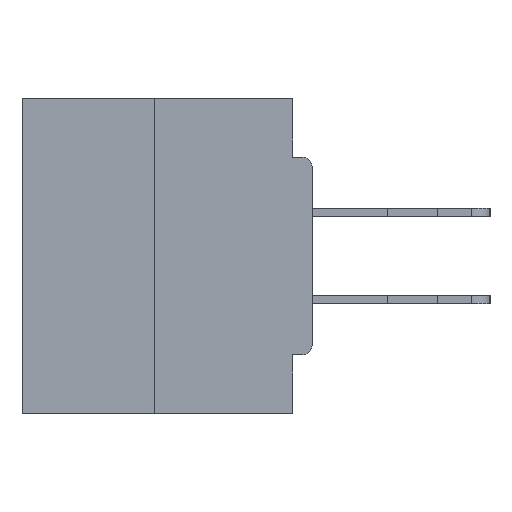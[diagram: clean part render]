
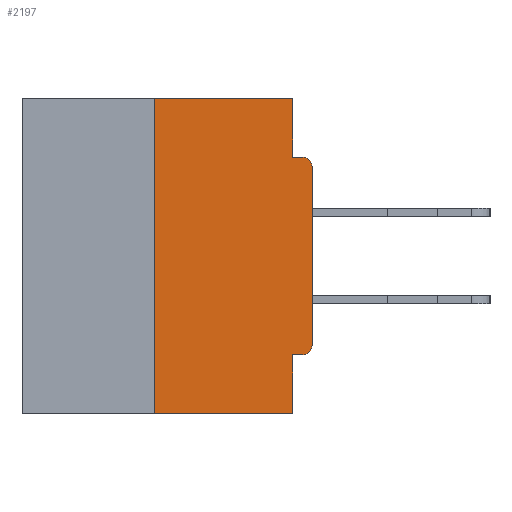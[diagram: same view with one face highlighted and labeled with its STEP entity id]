
A CAD part, left-side view. The second image highlights one B-rep face of the part: STEP entity #2197.
In plain terms, the highlighted planar face has unit normal (-1, 0, 0).
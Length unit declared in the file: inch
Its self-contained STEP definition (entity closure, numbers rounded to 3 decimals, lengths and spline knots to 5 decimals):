
#971 = EDGE_CURVE ( 'NONE', #14199, #31464, #19182, .T. ) ;
#2197 = ADVANCED_FACE ( 'NONE', ( #35479 ), #38009, .F. ) ;
#3407 = CARTESIAN_POINT ( 'NONE',  ( 0., 0.031, -0.0935 ) ) ;
#3553 = VECTOR ( 'NONE', #7746, 39.37008 ) ;
#3851 = VECTOR ( 'NONE', #30410, 39.37008 ) ;
#4221 = EDGE_CURVE ( 'NONE', #8972, #27702, #33297, .T. ) ;
#4298 = ORIENTED_EDGE ( 'NONE', *, *, #971, .F. ) ;
#4618 = DIRECTION ( 'NONE',  ( 0., 0., -1. ) ) ;
#4848 = LINE ( 'NONE', #19210, #3553 ) ;
#4918 = ORIENTED_EDGE ( 'NONE', *, *, #19758, .T. ) ;
#4962 = CARTESIAN_POINT ( 'NONE',  ( 0., 0.031, 0. ) ) ;
#5164 = CARTESIAN_POINT ( 'NONE',  ( 0., 0.031, -0.4065 ) ) ;
#5593 = CARTESIAN_POINT ( 'NONE',  ( 0., 0.25, 0. ) ) ;
#5896 = CIRCLE ( 'NONE', #18916, 0.015 ) ;
#7720 = LINE ( 'NONE', #33471, #34243 ) ;
#7746 = DIRECTION ( 'NONE',  ( 0., -1., 0. ) ) ;
#8311 = ORIENTED_EDGE ( 'NONE', *, *, #11387, .T. ) ;
#8922 = CARTESIAN_POINT ( 'NONE',  ( 0., 0., 0. ) ) ;
#8959 = DIRECTION ( 'NONE',  ( 0., 0., -1. ) ) ;
#8972 = VERTEX_POINT ( 'NONE', #3407 ) ;
#9197 = ORIENTED_EDGE ( 'NONE', *, *, #15629, .F. ) ;
#9233 = DIRECTION ( 'NONE',  ( 0., 0., -1. ) ) ;
#11081 = ORIENTED_EDGE ( 'NONE', *, *, #15918, .F. ) ;
#11387 = EDGE_CURVE ( 'NONE', #31196, #21611, #28861, .T. ) ;
#11734 = CARTESIAN_POINT ( 'NONE',  ( 0., 0.015, -0.3915 ) ) ;
#11804 = ORIENTED_EDGE ( 'NONE', *, *, #35500, .T. ) ;
#12277 = EDGE_LOOP ( 'NONE', ( #4298, #31679, #11804, #11081, #9197, #8311, #4918, #31915, #13639, #12369 ) ) ;
#12329 = CARTESIAN_POINT ( 'NONE',  ( 0., 0.031, -0.5 ) ) ;
#12369 = ORIENTED_EDGE ( 'NONE', *, *, #23183, .F. ) ;
#13639 = ORIENTED_EDGE ( 'NONE', *, *, #4221, .F. ) ;
#14172 = LINE ( 'NONE', #4962, #29891 ) ;
#14199 = VERTEX_POINT ( 'NONE', #35915 ) ;
#14446 = DIRECTION ( 'NONE',  ( 1., 0., 0. ) ) ;
#15157 = VERTEX_POINT ( 'NONE', #23891 ) ;
#15280 = LINE ( 'NONE', #5593, #30061 ) ;
#15539 = CARTESIAN_POINT ( 'NONE',  ( 0., 0.031, 0. ) ) ;
#15629 = EDGE_CURVE ( 'NONE', #31196, #32451, #7720, .T. ) ;
#15918 = EDGE_CURVE ( 'NONE', #32451, #15157, #27238, .T. ) ;
#16836 = DIRECTION ( 'NONE',  ( -1., 0., 0. ) ) ;
#17012 = DIRECTION ( 'NONE',  ( 0., 0., -1. ) ) ;
#18804 = DIRECTION ( 'NONE',  ( 0., -1., 0. ) ) ;
#18916 = AXIS2_PLACEMENT_3D ( 'NONE', #19770, #16836, #4618 ) ;
#19182 = LINE ( 'NONE', #22088, #34776 ) ;
#19210 = CARTESIAN_POINT ( 'NONE',  ( 0., 0.46, -0.5 ) ) ;
#19758 = EDGE_CURVE ( 'NONE', #21611, #27375, #30027, .T. ) ;
#19770 = CARTESIAN_POINT ( 'NONE',  ( 0., 0.015, -0.1085 ) ) ;
#20304 = DIRECTION ( 'NONE',  ( -1., 0., 0. ) ) ;
#20454 = CARTESIAN_POINT ( 'NONE',  ( 0., 0.46, 0. ) ) ;
#20788 = DIRECTION ( 'NONE',  ( 0., 0., 1. ) ) ;
#20930 = EDGE_CURVE ( 'NONE', #27497, #14199, #15280, .T. ) ;
#21106 = DIRECTION ( 'NONE',  ( 0., 0., 1. ) ) ;
#21611 = VERTEX_POINT ( 'NONE', #35227 ) ;
#21923 = EDGE_CURVE ( 'NONE', #27375, #27702, #5896, .T. ) ;
#22088 = CARTESIAN_POINT ( 'NONE',  ( 0., 0.46, 0. ) ) ;
#23183 = EDGE_CURVE ( 'NONE', #31464, #8972, #14172, .T. ) ;
#23280 = DIRECTION ( 'NONE',  ( 0., 0., -1. ) ) ;
#23848 = VECTOR ( 'NONE', #20788, 39.37008 ) ;
#23891 = CARTESIAN_POINT ( 'NONE',  ( 0., 0.031, -0.5 ) ) ;
#24542 = CARTESIAN_POINT ( 'NONE',  ( 0., 0.25, -0.5 ) ) ;
#27238 = LINE ( 'NONE', #12329, #29357 ) ;
#27375 = VERTEX_POINT ( 'NONE', #31910 ) ;
#27497 = VERTEX_POINT ( 'NONE', #24542 ) ;
#27702 = VERTEX_POINT ( 'NONE', #38228 ) ;
#28044 = AXIS2_PLACEMENT_3D ( 'NONE', #20454, #14446, #8959 ) ;
#28254 = DIRECTION ( 'NONE',  ( 0., 1., 0. ) ) ;
#28861 = CIRCLE ( 'NONE', #34421, 0.015 ) ;
#29357 = VECTOR ( 'NONE', #9233, 39.37008 ) ;
#29891 = VECTOR ( 'NONE', #23280, 39.37008 ) ;
#30027 = LINE ( 'NONE', #8922, #23848 ) ;
#30061 = VECTOR ( 'NONE', #21106, 39.37008 ) ;
#30410 = DIRECTION ( 'NONE',  ( 0., -1., 0. ) ) ;
#31196 = VERTEX_POINT ( 'NONE', #34527 ) ;
#31464 = VERTEX_POINT ( 'NONE', #15539 ) ;
#31679 = ORIENTED_EDGE ( 'NONE', *, *, #20930, .F. ) ;
#31910 = CARTESIAN_POINT ( 'NONE',  ( 0., 0., -0.1085 ) ) ;
#31915 = ORIENTED_EDGE ( 'NONE', *, *, #21923, .T. ) ;
#32451 = VERTEX_POINT ( 'NONE', #5164 ) ;
#33297 = LINE ( 'NONE', #36557, #3851 ) ;
#33471 = CARTESIAN_POINT ( 'NONE',  ( 0., 0., -0.4065 ) ) ;
#34243 = VECTOR ( 'NONE', #28254, 39.37008 ) ;
#34421 = AXIS2_PLACEMENT_3D ( 'NONE', #11734, #20304, #17012 ) ;
#34527 = CARTESIAN_POINT ( 'NONE',  ( 0., 0.015, -0.4065 ) ) ;
#34776 = VECTOR ( 'NONE', #18804, 39.37008 ) ;
#35227 = CARTESIAN_POINT ( 'NONE',  ( 0., 0., -0.3915 ) ) ;
#35479 = FACE_OUTER_BOUND ( 'NONE', #12277, .T. ) ;
#35500 = EDGE_CURVE ( 'NONE', #27497, #15157, #4848, .T. ) ;
#35915 = CARTESIAN_POINT ( 'NONE',  ( 0., 0.25, 0. ) ) ;
#36557 = CARTESIAN_POINT ( 'NONE',  ( 0., 0., -0.0935 ) ) ;
#38009 = PLANE ( 'NONE',  #28044 ) ;
#38228 = CARTESIAN_POINT ( 'NONE',  ( 0., 0.015, -0.0935 ) ) ;
